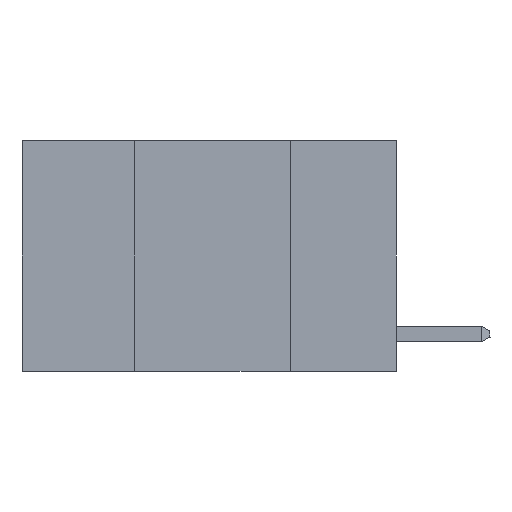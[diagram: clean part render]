
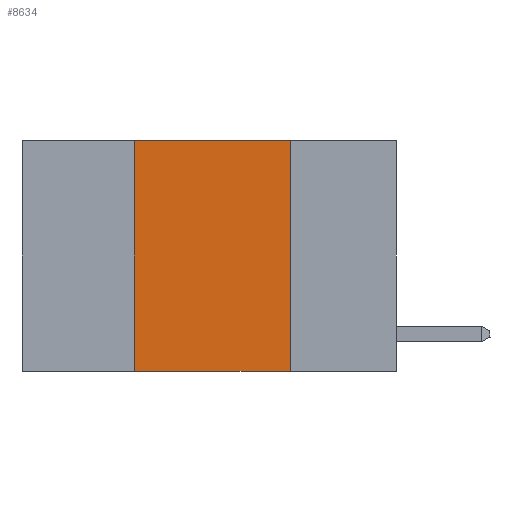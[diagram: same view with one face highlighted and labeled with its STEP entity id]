
A CAD part, left-side view. The second image highlights one B-rep face of the part: STEP entity #8634.
In plain terms, the highlighted planar face has unit normal (-1, 0, 0).
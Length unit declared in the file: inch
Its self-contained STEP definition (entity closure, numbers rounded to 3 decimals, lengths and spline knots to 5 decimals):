
#252 = VERTEX_POINT ( 'NONE', #7675 ) ;
#755 = EDGE_CURVE ( 'NONE', #3636, #11312, #13847, .T. ) ;
#932 = CARTESIAN_POINT ( 'NONE',  ( 0., 0.6, 0. ) ) ;
#1626 = EDGE_CURVE ( 'NONE', #252, #9736, #4968, .T. ) ;
#2439 = EDGE_CURVE ( 'NONE', #252, #3636, #10833, .T. ) ;
#2573 = VECTOR ( 'NONE', #9776, 39.37008 ) ;
#2699 = EDGE_CURVE ( 'NONE', #11312, #9736, #9106, .T. ) ;
#2713 = CARTESIAN_POINT ( 'NONE',  ( 0., 0.17, 0. ) ) ;
#2723 = CARTESIAN_POINT ( 'NONE',  ( 0., 0.17, -0.37 ) ) ;
#3636 = VERTEX_POINT ( 'NONE', #11390 ) ;
#3784 = DIRECTION ( 'NONE',  ( 0., 0., -1. ) ) ;
#3868 = VECTOR ( 'NONE', #13770, 39.37008 ) ;
#4016 = DIRECTION ( 'NONE',  ( 0., -1., 0. ) ) ;
#4091 = ORIENTED_EDGE ( 'NONE', *, *, #1626, .T. ) ;
#4879 = DIRECTION ( 'NONE',  ( 1., 0., 0. ) ) ;
#4968 = LINE ( 'NONE', #8234, #12246 ) ;
#5964 = PLANE ( 'NONE',  #13968 ) ;
#6106 = DIRECTION ( 'NONE',  ( 0., 0., -1. ) ) ;
#7675 = CARTESIAN_POINT ( 'NONE',  ( 0., 0.42, -0.37 ) ) ;
#8234 = CARTESIAN_POINT ( 'NONE',  ( 0., 0.6, -0.37 ) ) ;
#8634 = ADVANCED_FACE ( 'NONE', ( #11695 ), #5964, .F. ) ;
#9106 = LINE ( 'NONE', #2713, #11603 ) ;
#9337 = CARTESIAN_POINT ( 'NONE',  ( 0., 0.6, 0. ) ) ;
#9736 = VERTEX_POINT ( 'NONE', #2723 ) ;
#9776 = DIRECTION ( 'NONE',  ( 0., 0., 1. ) ) ;
#10833 = LINE ( 'NONE', #11908, #2573 ) ;
#11312 = VERTEX_POINT ( 'NONE', #11801 ) ;
#11390 = CARTESIAN_POINT ( 'NONE',  ( 0., 0.42, 0. ) ) ;
#11603 = VECTOR ( 'NONE', #3784, 39.37008 ) ;
#11695 = FACE_OUTER_BOUND ( 'NONE', #13342, .T. ) ;
#11721 = ORIENTED_EDGE ( 'NONE', *, *, #2439, .F. ) ;
#11801 = CARTESIAN_POINT ( 'NONE',  ( 0., 0.17, 0. ) ) ;
#11908 = CARTESIAN_POINT ( 'NONE',  ( 0., 0.42, 0. ) ) ;
#12246 = VECTOR ( 'NONE', #4016, 39.37008 ) ;
#12695 = ORIENTED_EDGE ( 'NONE', *, *, #755, .F. ) ;
#13342 = EDGE_LOOP ( 'NONE', ( #13695, #12695, #11721, #4091 ) ) ;
#13695 = ORIENTED_EDGE ( 'NONE', *, *, #2699, .F. ) ;
#13770 = DIRECTION ( 'NONE',  ( 0., -1., 0. ) ) ;
#13847 = LINE ( 'NONE', #932, #3868 ) ;
#13968 = AXIS2_PLACEMENT_3D ( 'NONE', #9337, #4879, #6106 ) ;
